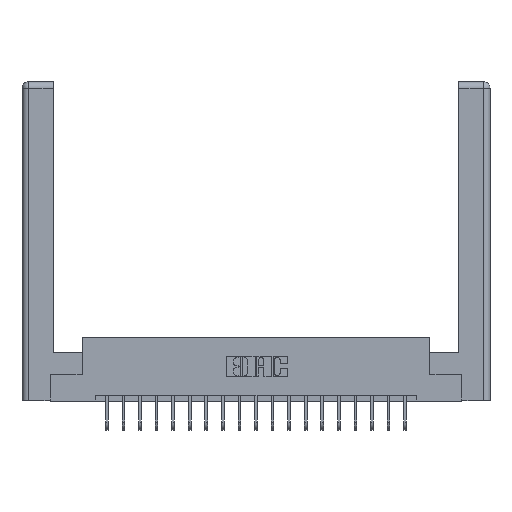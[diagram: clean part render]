
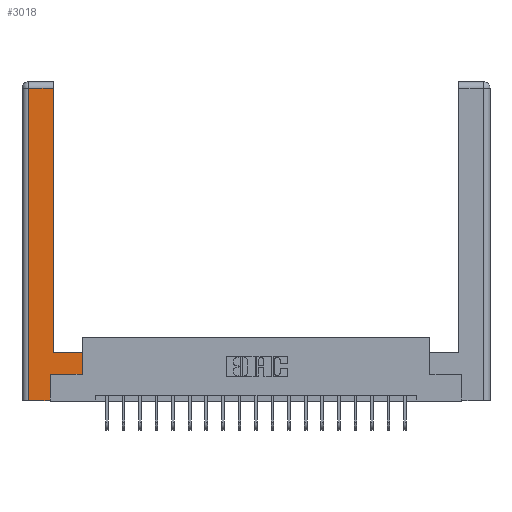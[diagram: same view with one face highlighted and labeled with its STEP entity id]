
A CAD part, top view. The second image highlights one B-rep face of the part: STEP entity #3018.
In plain terms, the highlighted planar face has unit normal (0, 0, 1).
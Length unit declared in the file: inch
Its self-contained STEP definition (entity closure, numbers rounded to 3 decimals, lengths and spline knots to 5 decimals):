
#37 = DIRECTION ( 'NONE',  ( -1., 0., 0. ) ) ;
#542 = CARTESIAN_POINT ( 'NONE',  ( 0.0615, 0., 0. ) ) ;
#580 = EDGE_CURVE ( 'NONE', #6254, #1903, #9329, .T. ) ;
#683 = VECTOR ( 'NONE', #21224, 39.37008 ) ;
#1259 = CARTESIAN_POINT ( 'NONE',  ( 0.265, 0., 0. ) ) ;
#1747 = LINE ( 'NONE', #11856, #2558 ) ;
#1903 = VERTEX_POINT ( 'NONE', #19497 ) ;
#2087 = VERTEX_POINT ( 'NONE', #542 ) ;
#2311 = DIRECTION ( 'NONE',  ( 0., 1., 0. ) ) ;
#2558 = VECTOR ( 'NONE', #15517, 39.37008 ) ;
#2918 = VERTEX_POINT ( 'NONE', #16497 ) ;
#3018 = ADVANCED_FACE ( 'NONE', ( #11865 ), #20515, .F. ) ;
#3750 = ORIENTED_EDGE ( 'NONE', *, *, #3865, .T. ) ;
#3751 = LINE ( 'NONE', #20510, #9601 ) ;
#3865 = EDGE_CURVE ( 'NONE', #4127, #6254, #7362, .T. ) ;
#4034 = CARTESIAN_POINT ( 'NONE',  ( 0.565, 0.45, 0. ) ) ;
#4127 = VERTEX_POINT ( 'NONE', #16980 ) ;
#4207 = EDGE_CURVE ( 'NONE', #2087, #4127, #11320, .T. ) ;
#5113 = EDGE_CURVE ( 'NONE', #6410, #5177, #11789, .T. ) ;
#5177 = VERTEX_POINT ( 'NONE', #17660 ) ;
#5205 = DIRECTION ( 'NONE',  ( 0., 0., -1. ) ) ;
#5609 = ORIENTED_EDGE ( 'NONE', *, *, #580, .T. ) ;
#5733 = VECTOR ( 'NONE', #6536, 39.37008 ) ;
#6254 = VERTEX_POINT ( 'NONE', #19484 ) ;
#6410 = VERTEX_POINT ( 'NONE', #13133 ) ;
#6536 = DIRECTION ( 'NONE',  ( 1., 0., 0. ) ) ;
#7098 = DIRECTION ( 'NONE',  ( -1., 0., 0. ) ) ;
#7202 = CARTESIAN_POINT ( 'NONE',  ( 0.565, 0.245, 0. ) ) ;
#7362 = LINE ( 'NONE', #19451, #13720 ) ;
#7508 = ORIENTED_EDGE ( 'NONE', *, *, #5113, .T. ) ;
#9329 = LINE ( 'NONE', #7202, #11183 ) ;
#9478 = EDGE_CURVE ( 'NONE', #21604, #2087, #17052, .T. ) ;
#9601 = VECTOR ( 'NONE', #37, 39.37008 ) ;
#11183 = VECTOR ( 'NONE', #18998, 39.37008 ) ;
#11320 = LINE ( 'NONE', #1259, #5733 ) ;
#11789 = LINE ( 'NONE', #16220, #16657 ) ;
#11856 = CARTESIAN_POINT ( 'NONE',  ( 0.295, 0.45, 0. ) ) ;
#11865 = FACE_OUTER_BOUND ( 'NONE', #13723, .T. ) ;
#12171 = ORIENTED_EDGE ( 'NONE', *, *, #19504, .T. ) ;
#12443 = DIRECTION ( 'NONE',  ( 0., 1., 0. ) ) ;
#13133 = CARTESIAN_POINT ( 'NONE',  ( 0.295, 0.45, 0. ) ) ;
#13720 = VECTOR ( 'NONE', #2311, 39.37008 ) ;
#13723 = EDGE_LOOP ( 'NONE', ( #7508, #12171, #15070, #20537, #3750, #5609, #19322, #17253 ) ) ;
#14276 = LINE ( 'NONE', #4034, #19922 ) ;
#15070 = ORIENTED_EDGE ( 'NONE', *, *, #9478, .T. ) ;
#15517 = DIRECTION ( 'NONE',  ( -1., 0., 0. ) ) ;
#15971 = DIRECTION ( 'NONE',  ( 0., 1., 0. ) ) ;
#16220 = CARTESIAN_POINT ( 'NONE',  ( 0.295, 3., 0. ) ) ;
#16497 = CARTESIAN_POINT ( 'NONE',  ( 0.565, 0.45, 0. ) ) ;
#16655 = EDGE_CURVE ( 'NONE', #2918, #6410, #1747, .T. ) ;
#16657 = VECTOR ( 'NONE', #12443, 39.37008 ) ;
#16980 = CARTESIAN_POINT ( 'NONE',  ( 0.265, 0., 0. ) ) ;
#16985 = EDGE_CURVE ( 'NONE', #1903, #2918, #14276, .T. ) ;
#17052 = LINE ( 'NONE', #19754, #683 ) ;
#17253 = ORIENTED_EDGE ( 'NONE', *, *, #16655, .T. ) ;
#17333 = CARTESIAN_POINT ( 'NONE',  ( 0., 0., 0. ) ) ;
#17660 = CARTESIAN_POINT ( 'NONE',  ( 0.295, 2.94, 0. ) ) ;
#18998 = DIRECTION ( 'NONE',  ( 1., 0., 0. ) ) ;
#19322 = ORIENTED_EDGE ( 'NONE', *, *, #16985, .T. ) ;
#19451 = CARTESIAN_POINT ( 'NONE',  ( 0.265, 0.245, 0. ) ) ;
#19484 = CARTESIAN_POINT ( 'NONE',  ( 0.265, 0.245, 0. ) ) ;
#19497 = CARTESIAN_POINT ( 'NONE',  ( 0.565, 0.245, 0. ) ) ;
#19504 = EDGE_CURVE ( 'NONE', #5177, #21604, #3751, .T. ) ;
#19754 = CARTESIAN_POINT ( 'NONE',  ( 0.0615, 0., 0. ) ) ;
#19922 = VECTOR ( 'NONE', #15971, 39.37008 ) ;
#20510 = CARTESIAN_POINT ( 'NONE',  ( 0.0615, 2.94, 0. ) ) ;
#20515 = PLANE ( 'NONE',  #20556 ) ;
#20537 = ORIENTED_EDGE ( 'NONE', *, *, #4207, .T. ) ;
#20556 = AXIS2_PLACEMENT_3D ( 'NONE', #17333, #5205, #7098 ) ;
#21173 = CARTESIAN_POINT ( 'NONE',  ( 0.0615, 2.94, 0. ) ) ;
#21224 = DIRECTION ( 'NONE',  ( 0., -1., 0. ) ) ;
#21604 = VERTEX_POINT ( 'NONE', #21173 ) ;
